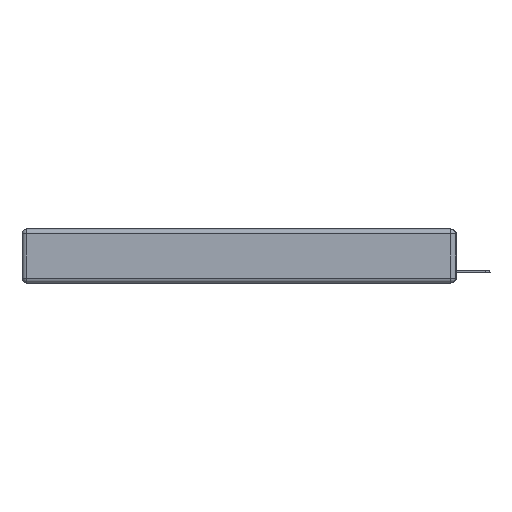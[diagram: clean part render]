
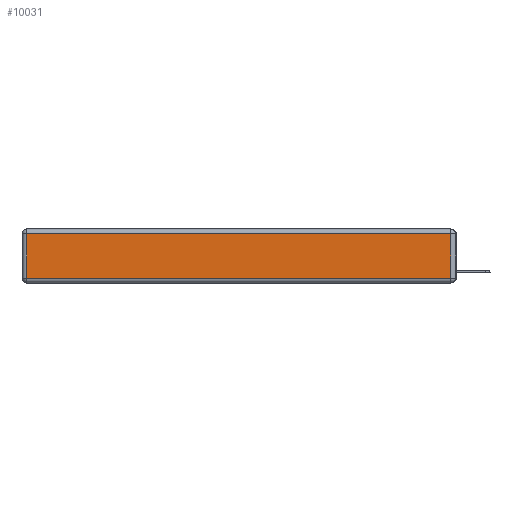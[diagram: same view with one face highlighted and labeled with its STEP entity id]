
A CAD part, left-side view. The second image highlights one B-rep face of the part: STEP entity #10031.
In plain terms, the highlighted planar face has unit normal (-1, 0, 0).
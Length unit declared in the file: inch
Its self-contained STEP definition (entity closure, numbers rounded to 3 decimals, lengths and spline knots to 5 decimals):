
#514 = VECTOR ( 'NONE', #11864, 39.37008 ) ;
#669 = CARTESIAN_POINT ( 'NONE',  ( 0., 2.75, -0.03 ) ) ;
#1460 = LINE ( 'NONE', #7631, #514 ) ;
#1656 = EDGE_LOOP ( 'NONE', ( #23913, #17161, #26520, #16733 ) ) ;
#2669 = VECTOR ( 'NONE', #16649, 39.37008 ) ;
#3523 = LINE ( 'NONE', #18979, #2669 ) ;
#5170 = CARTESIAN_POINT ( 'NONE',  ( 0., 2.72, -0.03 ) ) ;
#5427 = CARTESIAN_POINT ( 'NONE',  ( 0., 0., -0.343 ) ) ;
#6186 = CARTESIAN_POINT ( 'NONE',  ( 0., 2.72, -0.343 ) ) ;
#7559 = EDGE_CURVE ( 'NONE', #26306, #10334, #1460, .T. ) ;
#7566 = CARTESIAN_POINT ( 'NONE',  ( 0., 2.72, -0.313 ) ) ;
#7631 = CARTESIAN_POINT ( 'NONE',  ( 0., 0., -0.313 ) ) ;
#7882 = PLANE ( 'NONE',  #20735 ) ;
#8877 = LINE ( 'NONE', #669, #22347 ) ;
#10031 = ADVANCED_FACE ( 'NONE', ( #14177 ), #7882, .T. ) ;
#10059 = VECTOR ( 'NONE', #22492, 39.37008 ) ;
#10334 = VERTEX_POINT ( 'NONE', #13467 ) ;
#11864 = DIRECTION ( 'NONE',  ( 0., -1., 0. ) ) ;
#12817 = VERTEX_POINT ( 'NONE', #22758 ) ;
#13467 = CARTESIAN_POINT ( 'NONE',  ( 0., 0.03, -0.313 ) ) ;
#14177 = FACE_OUTER_BOUND ( 'NONE', #1656, .T. ) ;
#15162 = DIRECTION ( 'NONE',  ( 0., 1., 0. ) ) ;
#15284 = VERTEX_POINT ( 'NONE', #5170 ) ;
#16649 = DIRECTION ( 'NONE',  ( 0., 0., 1. ) ) ;
#16733 = ORIENTED_EDGE ( 'NONE', *, *, #20458, .T. ) ;
#17161 = ORIENTED_EDGE ( 'NONE', *, *, #21442, .T. ) ;
#18646 = LINE ( 'NONE', #6186, #10059 ) ;
#18979 = CARTESIAN_POINT ( 'NONE',  ( 0., 0.03, -0.343 ) ) ;
#20458 = EDGE_CURVE ( 'NONE', #15284, #26306, #18646, .T. ) ;
#20735 = AXIS2_PLACEMENT_3D ( 'NONE', #5427, #26668, #24053 ) ;
#21161 = EDGE_CURVE ( 'NONE', #12817, #15284, #8877, .T. ) ;
#21442 = EDGE_CURVE ( 'NONE', #10334, #12817, #3523, .T. ) ;
#22347 = VECTOR ( 'NONE', #15162, 39.37008 ) ;
#22492 = DIRECTION ( 'NONE',  ( 0., 0., -1. ) ) ;
#22758 = CARTESIAN_POINT ( 'NONE',  ( 0., 0.03, -0.03 ) ) ;
#23913 = ORIENTED_EDGE ( 'NONE', *, *, #7559, .T. ) ;
#24053 = DIRECTION ( 'NONE',  ( 0., 0., 1. ) ) ;
#26306 = VERTEX_POINT ( 'NONE', #7566 ) ;
#26520 = ORIENTED_EDGE ( 'NONE', *, *, #21161, .T. ) ;
#26668 = DIRECTION ( 'NONE',  ( -1., 0., 0. ) ) ;
